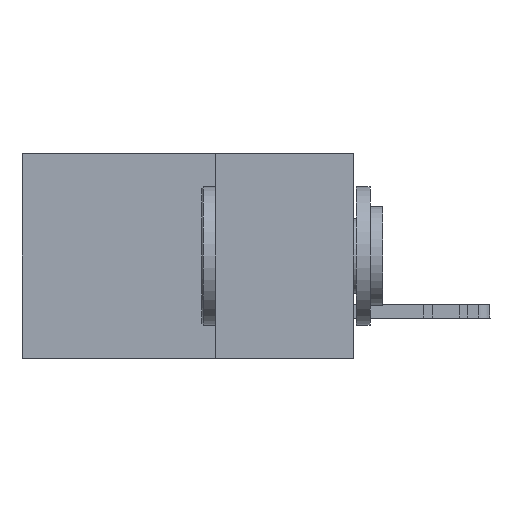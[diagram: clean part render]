
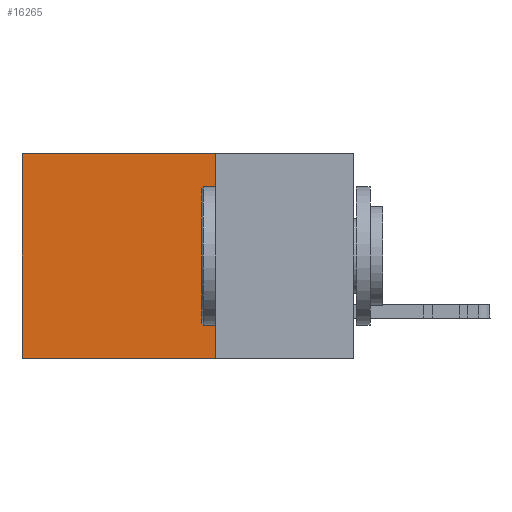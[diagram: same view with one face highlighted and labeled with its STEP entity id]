
A CAD part, left-side view. The second image highlights one B-rep face of the part: STEP entity #16265.
In plain terms, the highlighted planar face has unit normal (-1, 0, 0).
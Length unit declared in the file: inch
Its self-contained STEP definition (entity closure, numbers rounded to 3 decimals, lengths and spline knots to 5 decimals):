
#886 = AXIS2_PLACEMENT_3D ( 'NONE', #17164, #1612, #4491 ) ;
#1612 = DIRECTION ( 'NONE',  ( 1., 0., 0. ) ) ;
#1788 = VECTOR ( 'NONE', #32727, 39.37008 ) ;
#2329 = CARTESIAN_POINT ( 'NONE',  ( 0.2875, 0.6, 0. ) ) ;
#4491 = DIRECTION ( 'NONE',  ( 0., 0., -1. ) ) ;
#4945 = VERTEX_POINT ( 'NONE', #20022 ) ;
#6215 = DIRECTION ( 'NONE',  ( 0., 0., -1. ) ) ;
#10826 = CARTESIAN_POINT ( 'NONE',  ( 0.2875, 0.6, 0. ) ) ;
#12102 = EDGE_CURVE ( 'NONE', #25391, #39113, #16172, .T. ) ;
#12576 = ORIENTED_EDGE ( 'NONE', *, *, #12102, .T. ) ;
#12830 = FACE_OUTER_BOUND ( 'NONE', #23440, .T. ) ;
#13287 = EDGE_CURVE ( 'NONE', #25621, #4945, #15589, .T. ) ;
#13492 = CARTESIAN_POINT ( 'NONE',  ( 0.2875, 0.25, -0.37 ) ) ;
#15589 = LINE ( 'NONE', #26502, #1788 ) ;
#15868 = EDGE_CURVE ( 'NONE', #39113, #4945, #17305, .T. ) ;
#16172 = LINE ( 'NONE', #20676, #40848 ) ;
#16265 = ADVANCED_FACE ( 'NONE', ( #12830 ), #39788, .F. ) ;
#17164 = CARTESIAN_POINT ( 'NONE',  ( 0.2875, 0.25, 0. ) ) ;
#17305 = LINE ( 'NONE', #2329, #30149 ) ;
#19216 = ORIENTED_EDGE ( 'NONE', *, *, #15868, .T. ) ;
#20022 = CARTESIAN_POINT ( 'NONE',  ( 0.2875, 0.6, -0.37 ) ) ;
#20108 = ORIENTED_EDGE ( 'NONE', *, *, #13287, .F. ) ;
#20676 = CARTESIAN_POINT ( 'NONE',  ( 0.2875, 0.25, 0. ) ) ;
#21931 = DIRECTION ( 'NONE',  ( 0., 1., 0. ) ) ;
#22378 = ORIENTED_EDGE ( 'NONE', *, *, #26951, .F. ) ;
#22835 = VECTOR ( 'NONE', #6215, 39.37008 ) ;
#23440 = EDGE_LOOP ( 'NONE', ( #19216, #20108, #22378, #12576 ) ) ;
#25391 = VERTEX_POINT ( 'NONE', #30345 ) ;
#25621 = VERTEX_POINT ( 'NONE', #13492 ) ;
#26502 = CARTESIAN_POINT ( 'NONE',  ( 0.2875, 0.25, -0.37 ) ) ;
#26951 = EDGE_CURVE ( 'NONE', #25391, #25621, #35197, .T. ) ;
#27615 = CARTESIAN_POINT ( 'NONE',  ( 0.2875, 0.25, 0. ) ) ;
#27835 = DIRECTION ( 'NONE',  ( 0., 0., -1. ) ) ;
#30149 = VECTOR ( 'NONE', #27835, 39.37008 ) ;
#30345 = CARTESIAN_POINT ( 'NONE',  ( 0.2875, 0.25, 0. ) ) ;
#32727 = DIRECTION ( 'NONE',  ( 0., 1., 0. ) ) ;
#35197 = LINE ( 'NONE', #27615, #22835 ) ;
#39113 = VERTEX_POINT ( 'NONE', #10826 ) ;
#39788 = PLANE ( 'NONE',  #886 ) ;
#40848 = VECTOR ( 'NONE', #21931, 39.37008 ) ;
